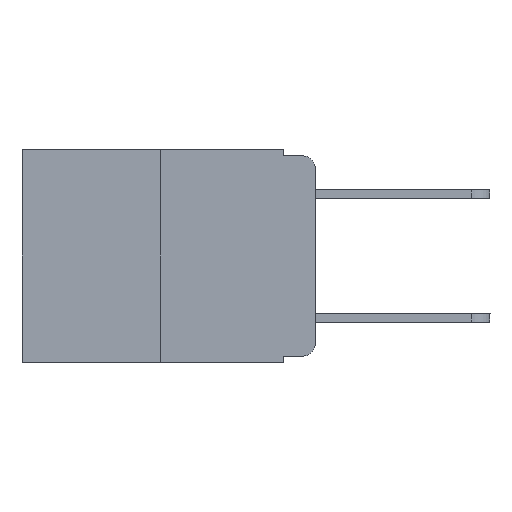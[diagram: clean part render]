
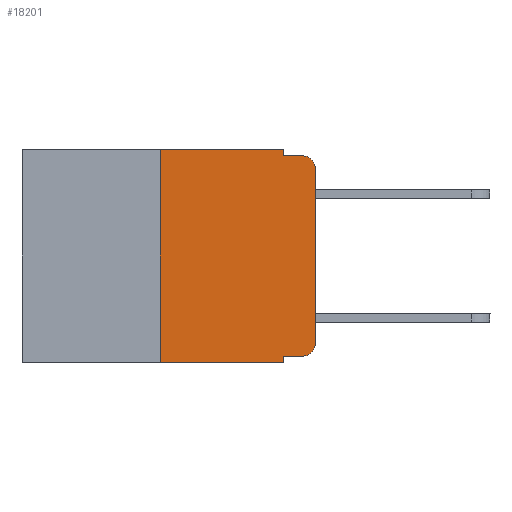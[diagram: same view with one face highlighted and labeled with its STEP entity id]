
A CAD part, left-side view. The second image highlights one B-rep face of the part: STEP entity #18201.
In plain terms, the highlighted planar face has unit normal (-1, 0, 0).
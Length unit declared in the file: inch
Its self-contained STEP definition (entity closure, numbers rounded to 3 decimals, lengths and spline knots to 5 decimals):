
#442 = LINE ( 'NONE', #17340, #3810 ) ;
#1040 = EDGE_CURVE ( 'NONE', #7155, #12483, #14499, .T. ) ;
#1246 = ORIENTED_EDGE ( 'NONE', *, *, #9800, .T. ) ;
#1543 = EDGE_CURVE ( 'NONE', #5452, #15345, #2702, .T. ) ;
#1705 = LINE ( 'NONE', #14478, #9407 ) ;
#2158 = VERTEX_POINT ( 'NONE', #15231 ) ;
#2370 = CARTESIAN_POINT ( 'NONE',  ( 0., 0.25, 0. ) ) ;
#2686 = FACE_OUTER_BOUND ( 'NONE', #19707, .T. ) ;
#2702 = LINE ( 'NONE', #2370, #13211 ) ;
#2729 = EDGE_CURVE ( 'NONE', #5452, #13849, #4437, .T. ) ;
#3054 = ORIENTED_EDGE ( 'NONE', *, *, #1040, .F. ) ;
#3217 = LINE ( 'NONE', #10418, #19345 ) ;
#3446 = EDGE_CURVE ( 'NONE', #16466, #12483, #15159, .T. ) ;
#3560 = CARTESIAN_POINT ( 'NONE',  ( 0., 0.02, -0.01 ) ) ;
#3810 = VECTOR ( 'NONE', #14195, 39.37008 ) ;
#4437 = LINE ( 'NONE', #11621, #10574 ) ;
#4524 = CARTESIAN_POINT ( 'NONE',  ( 0., 0.02, -0.03 ) ) ;
#4621 = CARTESIAN_POINT ( 'NONE',  ( 0., 0.473, 0. ) ) ;
#4711 = DIRECTION ( 'NONE',  ( 0., -1., 0. ) ) ;
#5292 = ORIENTED_EDGE ( 'NONE', *, *, #3446, .T. ) ;
#5452 = VERTEX_POINT ( 'NONE', #6549 ) ;
#5736 = DIRECTION ( 'NONE',  ( 0., 0., 1. ) ) ;
#5751 = CARTESIAN_POINT ( 'NONE',  ( 0., 0.051, -0.333 ) ) ;
#5813 = ORIENTED_EDGE ( 'NONE', *, *, #15755, .F. ) ;
#6104 = PLANE ( 'NONE',  #11620 ) ;
#6419 = CARTESIAN_POINT ( 'NONE',  ( 0., 0.051, -0.01 ) ) ;
#6470 = EDGE_CURVE ( 'NONE', #16773, #16466, #1705, .T. ) ;
#6496 = CARTESIAN_POINT ( 'NONE',  ( 0., 0.02, -0.313 ) ) ;
#6549 = CARTESIAN_POINT ( 'NONE',  ( 0., 0.25, -0.343 ) ) ;
#7155 = VERTEX_POINT ( 'NONE', #15461 ) ;
#7465 = VECTOR ( 'NONE', #7599, 39.37008 ) ;
#7599 = DIRECTION ( 'NONE',  ( 0., -1., 0. ) ) ;
#8188 = CARTESIAN_POINT ( 'NONE',  ( 0., 0., -0.03 ) ) ;
#8495 = DIRECTION ( 'NONE',  ( 0., -1., 0. ) ) ;
#9407 = VECTOR ( 'NONE', #11167, 39.37008 ) ;
#9760 = DIRECTION ( 'NONE',  ( 0., 0., -1. ) ) ;
#9800 = EDGE_CURVE ( 'NONE', #19964, #16773, #18912, .T. ) ;
#9935 = LINE ( 'NONE', #4621, #13801 ) ;
#10418 = CARTESIAN_POINT ( 'NONE',  ( 0., 0.051, 0. ) ) ;
#10536 = EDGE_CURVE ( 'NONE', #2158, #7155, #3217, .T. ) ;
#10574 = VECTOR ( 'NONE', #8495, 39.37008 ) ;
#10811 = CARTESIAN_POINT ( 'NONE',  ( 0., 0.051, -0.343 ) ) ;
#11167 = DIRECTION ( 'NONE',  ( 0., 0., 1. ) ) ;
#11184 = CARTESIAN_POINT ( 'NONE',  ( 0., 0.25, 0. ) ) ;
#11226 = ORIENTED_EDGE ( 'NONE', *, *, #2729, .T. ) ;
#11620 = AXIS2_PLACEMENT_3D ( 'NONE', #12894, #12814, #15878 ) ;
#11621 = CARTESIAN_POINT ( 'NONE',  ( 0., 0.473, -0.343 ) ) ;
#12294 = CARTESIAN_POINT ( 'NONE',  ( 0., 0., -0.313 ) ) ;
#12483 = VERTEX_POINT ( 'NONE', #3560 ) ;
#12568 = CARTESIAN_POINT ( 'NONE',  ( 0., 0.051, -0.333 ) ) ;
#12814 = DIRECTION ( 'NONE',  ( 1., 0., 0. ) ) ;
#12815 = DIRECTION ( 'NONE',  ( 0., 0., -1. ) ) ;
#12894 = CARTESIAN_POINT ( 'NONE',  ( 0., 0.473, 0. ) ) ;
#12985 = ORIENTED_EDGE ( 'NONE', *, *, #10536, .F. ) ;
#13211 = VECTOR ( 'NONE', #5736, 39.37008 ) ;
#13350 = AXIS2_PLACEMENT_3D ( 'NONE', #4524, #20766, #12815 ) ;
#13367 = ORIENTED_EDGE ( 'NONE', *, *, #14549, .T. ) ;
#13392 = ORIENTED_EDGE ( 'NONE', *, *, #6470, .T. ) ;
#13656 = DIRECTION ( 'NONE',  ( 0., 0., -1. ) ) ;
#13801 = VECTOR ( 'NONE', #17779, 39.37008 ) ;
#13849 = VERTEX_POINT ( 'NONE', #10811 ) ;
#14195 = DIRECTION ( 'NONE',  ( 0., 0., -1. ) ) ;
#14478 = CARTESIAN_POINT ( 'NONE',  ( 0., 0., 0. ) ) ;
#14499 = LINE ( 'NONE', #6419, #17307 ) ;
#14549 = EDGE_CURVE ( 'NONE', #18066, #19964, #17681, .T. ) ;
#15159 = CIRCLE ( 'NONE', #13350, 0.02 ) ;
#15231 = CARTESIAN_POINT ( 'NONE',  ( 0., 0.051, 0. ) ) ;
#15345 = VERTEX_POINT ( 'NONE', #11184 ) ;
#15437 = EDGE_CURVE ( 'NONE', #15345, #2158, #9935, .T. ) ;
#15461 = CARTESIAN_POINT ( 'NONE',  ( 0., 0.051, -0.01 ) ) ;
#15755 = EDGE_CURVE ( 'NONE', #18066, #13849, #442, .T. ) ;
#15878 = DIRECTION ( 'NONE',  ( 0., 0., -1. ) ) ;
#15946 = ORIENTED_EDGE ( 'NONE', *, *, #15437, .F. ) ;
#16466 = VERTEX_POINT ( 'NONE', #8188 ) ;
#16773 = VERTEX_POINT ( 'NONE', #12294 ) ;
#17307 = VECTOR ( 'NONE', #4711, 39.37008 ) ;
#17340 = CARTESIAN_POINT ( 'NONE',  ( 0., 0.051, 0. ) ) ;
#17483 = ORIENTED_EDGE ( 'NONE', *, *, #1543, .F. ) ;
#17681 = LINE ( 'NONE', #12568, #7465 ) ;
#17779 = DIRECTION ( 'NONE',  ( 0., -1., 0. ) ) ;
#17949 = AXIS2_PLACEMENT_3D ( 'NONE', #6496, #19586, #9760 ) ;
#18066 = VERTEX_POINT ( 'NONE', #5751 ) ;
#18201 = ADVANCED_FACE ( 'NONE', ( #2686 ), #6104, .F. ) ;
#18912 = CIRCLE ( 'NONE', #17949, 0.02 ) ;
#19345 = VECTOR ( 'NONE', #13656, 39.37008 ) ;
#19379 = CARTESIAN_POINT ( 'NONE',  ( 0., 0.02, -0.333 ) ) ;
#19586 = DIRECTION ( 'NONE',  ( -1., 0., 0. ) ) ;
#19707 = EDGE_LOOP ( 'NONE', ( #13392, #5292, #3054, #12985, #15946, #17483, #11226, #5813, #13367, #1246 ) ) ;
#19964 = VERTEX_POINT ( 'NONE', #19379 ) ;
#20766 = DIRECTION ( 'NONE',  ( -1., 0., 0. ) ) ;
